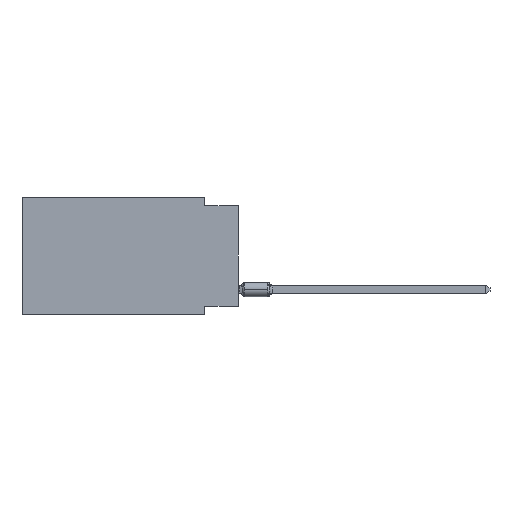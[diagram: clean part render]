
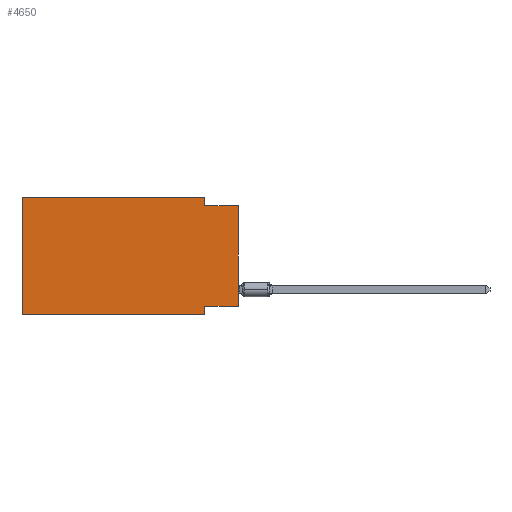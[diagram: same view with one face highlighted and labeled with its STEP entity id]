
A CAD part, left-side view. The second image highlights one B-rep face of the part: STEP entity #4650.
In plain terms, the highlighted planar face has unit normal (-1, 0, 0).
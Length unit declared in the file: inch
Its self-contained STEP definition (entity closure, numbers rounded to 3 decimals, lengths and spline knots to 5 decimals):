
#157 = EDGE_CURVE ( 'NONE', #8745, #10573, #11386, .T. ) ;
#186 = DIRECTION ( 'NONE',  ( 0., 1., 0. ) ) ;
#530 = ORIENTED_EDGE ( 'NONE', *, *, #8924, .F. ) ;
#559 = EDGE_CURVE ( 'NONE', #8745, #7012, #797, .T. ) ;
#587 = VECTOR ( 'NONE', #186, 39.37008 ) ;
#781 = ORIENTED_EDGE ( 'NONE', *, *, #157, .F. ) ;
#797 = LINE ( 'NONE', #8273, #8114 ) ;
#1320 = EDGE_LOOP ( 'NONE', ( #8586, #9711, #7627, #12948, #781, #11980, #10369, #530 ) ) ;
#2003 = VERTEX_POINT ( 'NONE', #7230 ) ;
#2121 = LINE ( 'NONE', #8193, #8589 ) ;
#2226 = CARTESIAN_POINT ( 'NONE',  ( 0., 0.1, -0.025 ) ) ;
#2536 = EDGE_CURVE ( 'NONE', #5848, #7012, #3200, .T. ) ;
#2540 = FACE_OUTER_BOUND ( 'NONE', #1320, .T. ) ;
#2608 = DIRECTION ( 'NONE',  ( 0., 0., -1. ) ) ;
#2997 = CARTESIAN_POINT ( 'NONE',  ( 0., 0.645, 0. ) ) ;
#3200 = LINE ( 'NONE', #5448, #10607 ) ;
#3227 = CARTESIAN_POINT ( 'NONE',  ( 0., 0.645, 0. ) ) ;
#3476 = CARTESIAN_POINT ( 'NONE',  ( 0., 0.1, 0. ) ) ;
#3630 = CARTESIAN_POINT ( 'NONE',  ( 0., 0.645, 0. ) ) ;
#3838 = DIRECTION ( 'NONE',  ( 0., -1., 0. ) ) ;
#4650 = ADVANCED_FACE ( 'NONE', ( #2540 ), #10805, .F. ) ;
#4928 = VECTOR ( 'NONE', #12212, 39.37008 ) ;
#4952 = DIRECTION ( 'NONE',  ( 0., -1., 0. ) ) ;
#4991 = VECTOR ( 'NONE', #3838, 39.37008 ) ;
#5448 = CARTESIAN_POINT ( 'NONE',  ( 0., 0.1, -0.35 ) ) ;
#5848 = VERTEX_POINT ( 'NONE', #13361 ) ;
#5975 = CARTESIAN_POINT ( 'NONE',  ( 0., 0.1, 0. ) ) ;
#6113 = DIRECTION ( 'NONE',  ( 0., -1., 0. ) ) ;
#6153 = DIRECTION ( 'NONE',  ( 0., 0., 1. ) ) ;
#6751 = LINE ( 'NONE', #7770, #9728 ) ;
#7012 = VERTEX_POINT ( 'NONE', #7035 ) ;
#7035 = CARTESIAN_POINT ( 'NONE',  ( 0., 0.1, -0.35 ) ) ;
#7076 = EDGE_CURVE ( 'NONE', #10833, #2003, #2121, .T. ) ;
#7230 = CARTESIAN_POINT ( 'NONE',  ( 0., 0., -0.025 ) ) ;
#7454 = CARTESIAN_POINT ( 'NONE',  ( 0., 0., -0.325 ) ) ;
#7627 = ORIENTED_EDGE ( 'NONE', *, *, #8722, .F. ) ;
#7770 = CARTESIAN_POINT ( 'NONE',  ( 0., 0., -0.025 ) ) ;
#8114 = VECTOR ( 'NONE', #4952, 39.37008 ) ;
#8148 = CARTESIAN_POINT ( 'NONE',  ( 0., 0.645, -0.35 ) ) ;
#8173 = LINE ( 'NONE', #2997, #4991 ) ;
#8193 = CARTESIAN_POINT ( 'NONE',  ( 0., 0., 0. ) ) ;
#8273 = CARTESIAN_POINT ( 'NONE',  ( 0., 0.645, -0.35 ) ) ;
#8586 = ORIENTED_EDGE ( 'NONE', *, *, #7076, .T. ) ;
#8589 = VECTOR ( 'NONE', #6153, 39.37008 ) ;
#8722 = EDGE_CURVE ( 'NONE', #12223, #11404, #8973, .T. ) ;
#8745 = VERTEX_POINT ( 'NONE', #8148 ) ;
#8924 = EDGE_CURVE ( 'NONE', #10833, #5848, #9376, .T. ) ;
#8973 = LINE ( 'NONE', #5975, #12540 ) ;
#9241 = DIRECTION ( 'NONE',  ( 0., 0., -1. ) ) ;
#9376 = LINE ( 'NONE', #7454, #587 ) ;
#9711 = ORIENTED_EDGE ( 'NONE', *, *, #9970, .F. ) ;
#9728 = VECTOR ( 'NONE', #6113, 39.37008 ) ;
#9970 = EDGE_CURVE ( 'NONE', #11404, #2003, #6751, .T. ) ;
#10175 = CARTESIAN_POINT ( 'NONE',  ( 0., 0., -0.325 ) ) ;
#10369 = ORIENTED_EDGE ( 'NONE', *, *, #2536, .F. ) ;
#10427 = CARTESIAN_POINT ( 'NONE',  ( 0., 0.645, 0. ) ) ;
#10573 = VERTEX_POINT ( 'NONE', #3227 ) ;
#10607 = VECTOR ( 'NONE', #12614, 39.37008 ) ;
#10805 = PLANE ( 'NONE',  #12489 ) ;
#10833 = VERTEX_POINT ( 'NONE', #10175 ) ;
#11386 = LINE ( 'NONE', #10427, #4928 ) ;
#11404 = VERTEX_POINT ( 'NONE', #2226 ) ;
#11828 = DIRECTION ( 'NONE',  ( 1., 0., 0. ) ) ;
#11980 = ORIENTED_EDGE ( 'NONE', *, *, #559, .T. ) ;
#12212 = DIRECTION ( 'NONE',  ( 0., 0., 1. ) ) ;
#12223 = VERTEX_POINT ( 'NONE', #3476 ) ;
#12463 = EDGE_CURVE ( 'NONE', #10573, #12223, #8173, .T. ) ;
#12489 = AXIS2_PLACEMENT_3D ( 'NONE', #3630, #11828, #2608 ) ;
#12540 = VECTOR ( 'NONE', #9241, 39.37008 ) ;
#12614 = DIRECTION ( 'NONE',  ( 0., 0., -1. ) ) ;
#12948 = ORIENTED_EDGE ( 'NONE', *, *, #12463, .F. ) ;
#13361 = CARTESIAN_POINT ( 'NONE',  ( 0., 0.1, -0.325 ) ) ;
